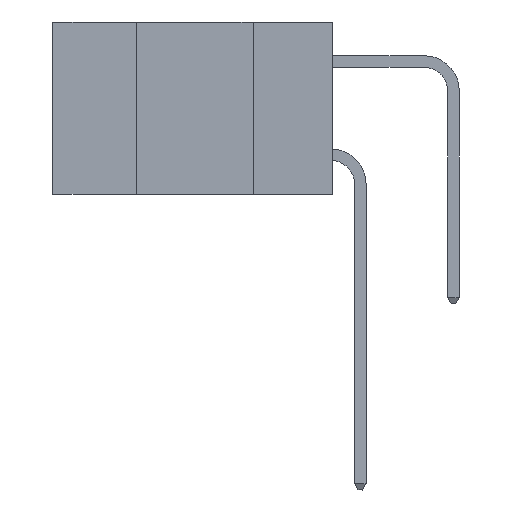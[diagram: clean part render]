
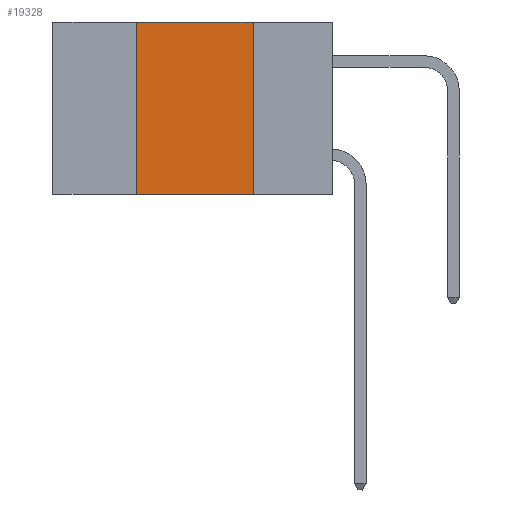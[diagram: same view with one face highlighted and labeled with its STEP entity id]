
A CAD part, left-side view. The second image highlights one B-rep face of the part: STEP entity #19328.
In plain terms, the highlighted planar face has unit normal (-1, 0, 0).
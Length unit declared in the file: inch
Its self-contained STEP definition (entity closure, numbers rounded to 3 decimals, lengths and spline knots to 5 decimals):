
#1292 = CARTESIAN_POINT ( 'NONE',  ( 0., 0.42, 0. ) ) ;
#1618 = FACE_OUTER_BOUND ( 'NONE', #16075, .T. ) ;
#1946 = CARTESIAN_POINT ( 'NONE',  ( 0., 0.6, -0.37 ) ) ;
#2592 = LINE ( 'NONE', #8346, #15843 ) ;
#3157 = VECTOR ( 'NONE', #6159, 39.37008 ) ;
#3799 = EDGE_CURVE ( 'NONE', #4231, #8767, #17002, .T. ) ;
#4231 = VERTEX_POINT ( 'NONE', #21239 ) ;
#5550 = VERTEX_POINT ( 'NONE', #11661 ) ;
#5936 = AXIS2_PLACEMENT_3D ( 'NONE', #6548, #18709, #8300 ) ;
#6159 = DIRECTION ( 'NONE',  ( 0., -1., 0. ) ) ;
#6548 = CARTESIAN_POINT ( 'NONE',  ( 0., 0.6, 0. ) ) ;
#7030 = ORIENTED_EDGE ( 'NONE', *, *, #21532, .F. ) ;
#8300 = DIRECTION ( 'NONE',  ( 0., 0., -1. ) ) ;
#8346 = CARTESIAN_POINT ( 'NONE',  ( 0., 0.42, 0. ) ) ;
#8618 = CARTESIAN_POINT ( 'NONE',  ( 0., 0.17, 0. ) ) ;
#8767 = VERTEX_POINT ( 'NONE', #20588 ) ;
#8838 = LINE ( 'NONE', #21542, #14011 ) ;
#9537 = DIRECTION ( 'NONE',  ( 0., -1., 0. ) ) ;
#10094 = DIRECTION ( 'NONE',  ( 0., 0., 1. ) ) ;
#11661 = CARTESIAN_POINT ( 'NONE',  ( 0., 0.17, 0. ) ) ;
#12485 = ORIENTED_EDGE ( 'NONE', *, *, #20433, .F. ) ;
#13080 = VERTEX_POINT ( 'NONE', #1292 ) ;
#13866 = DIRECTION ( 'NONE',  ( 0., 0., -1. ) ) ;
#13952 = VECTOR ( 'NONE', #13866, 39.37008 ) ;
#14011 = VECTOR ( 'NONE', #9537, 39.37008 ) ;
#14407 = ORIENTED_EDGE ( 'NONE', *, *, #3799, .T. ) ;
#15843 = VECTOR ( 'NONE', #10094, 39.37008 ) ;
#16075 = EDGE_LOOP ( 'NONE', ( #12485, #16716, #7030, #14407 ) ) ;
#16716 = ORIENTED_EDGE ( 'NONE', *, *, #19179, .F. ) ;
#17002 = LINE ( 'NONE', #1946, #3157 ) ;
#17012 = PLANE ( 'NONE',  #5936 ) ;
#18559 = LINE ( 'NONE', #8618, #13952 ) ;
#18709 = DIRECTION ( 'NONE',  ( 1., 0., 0. ) ) ;
#19179 = EDGE_CURVE ( 'NONE', #13080, #5550, #8838, .T. ) ;
#19328 = ADVANCED_FACE ( 'NONE', ( #1618 ), #17012, .F. ) ;
#20433 = EDGE_CURVE ( 'NONE', #5550, #8767, #18559, .T. ) ;
#20588 = CARTESIAN_POINT ( 'NONE',  ( 0., 0.17, -0.37 ) ) ;
#21239 = CARTESIAN_POINT ( 'NONE',  ( 0., 0.42, -0.37 ) ) ;
#21532 = EDGE_CURVE ( 'NONE', #4231, #13080, #2592, .T. ) ;
#21542 = CARTESIAN_POINT ( 'NONE',  ( 0., 0.6, 0. ) ) ;
